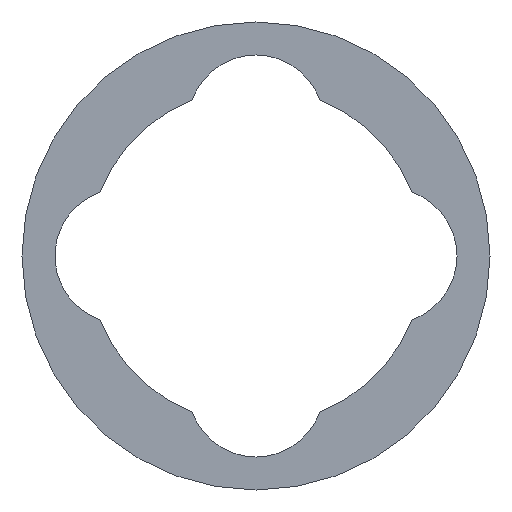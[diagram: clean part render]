
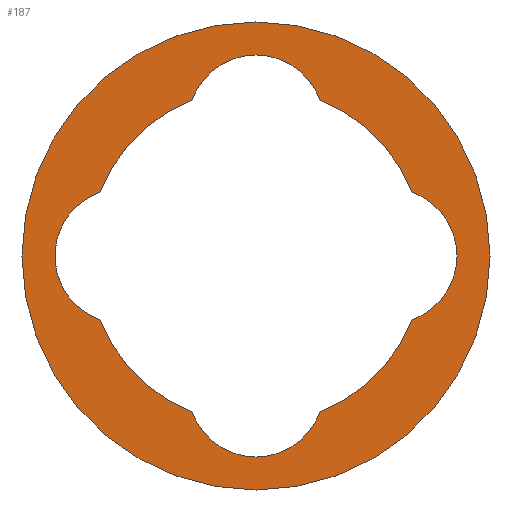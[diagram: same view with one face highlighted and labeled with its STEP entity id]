
A CAD part, front view. The second image highlights one B-rep face of the part: STEP entity #187.
In plain terms, the highlighted planar face has unit normal (0, -1, 0).
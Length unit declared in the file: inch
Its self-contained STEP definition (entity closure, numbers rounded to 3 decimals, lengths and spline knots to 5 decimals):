
#42=FACE_BOUND('',#56,.T.);
#44=FACE_OUTER_BOUND('',#55,.T.);
#55=EDGE_LOOP('',(#131));
#56=EDGE_LOOP('',(#132,#133,#134,#135,#136,#137,#138,#139));
#68=CIRCLE('',#219,0.17323);
#69=CIRCLE('',#220,0.05);
#70=CIRCLE('',#221,0.125);
#71=CIRCLE('',#222,0.05);
#72=CIRCLE('',#223,0.125);
#73=CIRCLE('',#224,0.05);
#74=CIRCLE('',#225,0.125);
#75=CIRCLE('',#226,0.05);
#76=CIRCLE('',#227,0.125);
#86=VERTEX_POINT('',#318);
#87=VERTEX_POINT('',#320);
#88=VERTEX_POINT('',#321);
#89=VERTEX_POINT('',#323);
#90=VERTEX_POINT('',#325);
#91=VERTEX_POINT('',#327);
#92=VERTEX_POINT('',#329);
#93=VERTEX_POINT('',#331);
#94=VERTEX_POINT('',#333);
#104=EDGE_CURVE('',#86,#86,#68,.T.);
#105=EDGE_CURVE('',#87,#88,#69,.T.);
#106=EDGE_CURVE('',#89,#87,#70,.T.);
#107=EDGE_CURVE('',#90,#89,#71,.T.);
#108=EDGE_CURVE('',#91,#90,#72,.T.);
#109=EDGE_CURVE('',#92,#91,#73,.T.);
#110=EDGE_CURVE('',#93,#92,#74,.T.);
#111=EDGE_CURVE('',#94,#93,#75,.T.);
#112=EDGE_CURVE('',#88,#94,#76,.T.);
#131=ORIENTED_EDGE('',*,*,#104,.F.);
#132=ORIENTED_EDGE('',*,*,#105,.F.);
#133=ORIENTED_EDGE('',*,*,#106,.F.);
#134=ORIENTED_EDGE('',*,*,#107,.F.);
#135=ORIENTED_EDGE('',*,*,#108,.F.);
#136=ORIENTED_EDGE('',*,*,#109,.F.);
#137=ORIENTED_EDGE('',*,*,#110,.F.);
#138=ORIENTED_EDGE('',*,*,#111,.F.);
#139=ORIENTED_EDGE('',*,*,#112,.F.);
#185=PLANE('',#218);
#187=ADVANCED_FACE('',(#44,#42),#185,.F.);
#218=AXIS2_PLACEMENT_3D('',#317,#249,#250);
#219=AXIS2_PLACEMENT_3D('',#319,#251,#252);
#220=AXIS2_PLACEMENT_3D('',#322,#253,#254);
#221=AXIS2_PLACEMENT_3D('',#324,#255,#256);
#222=AXIS2_PLACEMENT_3D('',#326,#257,#258);
#223=AXIS2_PLACEMENT_3D('',#328,#259,#260);
#224=AXIS2_PLACEMENT_3D('',#330,#261,#262);
#225=AXIS2_PLACEMENT_3D('',#332,#263,#264);
#226=AXIS2_PLACEMENT_3D('',#334,#265,#266);
#227=AXIS2_PLACEMENT_3D('',#335,#267,#268);
#249=DIRECTION('center_axis',(0.,1.,0.));
#250=DIRECTION('ref_axis',(0.,0.,1.));
#251=DIRECTION('center_axis',(0.,1.,0.));
#252=DIRECTION('ref_axis',(-1.,0.,0.));
#253=DIRECTION('center_axis',(0.,-1.,0.));
#254=DIRECTION('ref_axis',(-1.,0.,0.));
#255=DIRECTION('center_axis',(0.,-1.,0.));
#256=DIRECTION('ref_axis',(-1.,0.,0.));
#257=DIRECTION('center_axis',(0.,-1.,0.));
#258=DIRECTION('ref_axis',(-1.,0.,0.));
#259=DIRECTION('center_axis',(0.,-1.,0.));
#260=DIRECTION('ref_axis',(-1.,0.,0.));
#261=DIRECTION('center_axis',(0.,-1.,0.));
#262=DIRECTION('ref_axis',(-1.,0.,0.));
#263=DIRECTION('center_axis',(0.,-1.,0.));
#264=DIRECTION('ref_axis',(-1.,0.,0.));
#265=DIRECTION('center_axis',(0.,-1.,0.));
#266=DIRECTION('ref_axis',(-1.,0.,0.));
#267=DIRECTION('center_axis',(0.,-1.,0.));
#268=DIRECTION('ref_axis',(-1.,0.,0.));
#317=CARTESIAN_POINT('Origin',(0.,1.,0.));
#318=CARTESIAN_POINT('',(0.17323,1.,0.));
#319=CARTESIAN_POINT('Origin',(0.,1.,0.));
#320=CARTESIAN_POINT('',(0.04702,1.,0.11582));
#321=CARTESIAN_POINT('',(-0.04702,1.,0.11582));
#322=CARTESIAN_POINT('Origin',(0.,1.,0.09881));
#323=CARTESIAN_POINT('',(0.11582,1.,0.04702));
#324=CARTESIAN_POINT('Origin',(0.,1.,0.));
#325=CARTESIAN_POINT('',(0.11582,1.,-0.04702));
#326=CARTESIAN_POINT('Origin',(0.09881,1.,0.));
#327=CARTESIAN_POINT('',(0.04702,1.,-0.11582));
#328=CARTESIAN_POINT('Origin',(0.,1.,0.));
#329=CARTESIAN_POINT('',(-0.04702,1.,-0.11582));
#330=CARTESIAN_POINT('Origin',(0.,1.,-0.09881));
#331=CARTESIAN_POINT('',(-0.11581,1.,-0.04704));
#332=CARTESIAN_POINT('Origin',(0.,1.,0.));
#333=CARTESIAN_POINT('',(-0.11581,1.,0.04704));
#334=CARTESIAN_POINT('Origin',(-0.09887,1.,0.));
#335=CARTESIAN_POINT('Origin',(0.,1.,0.));
